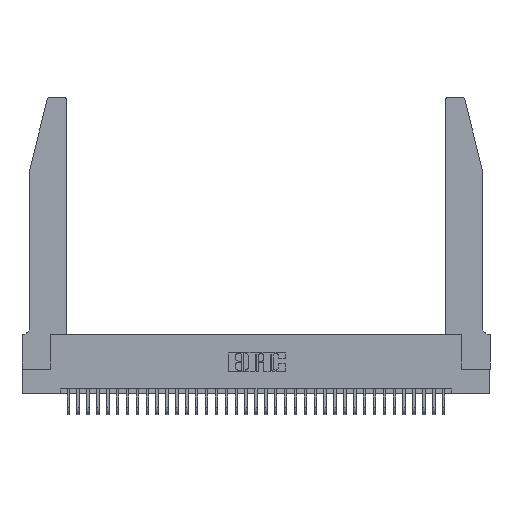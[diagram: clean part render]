
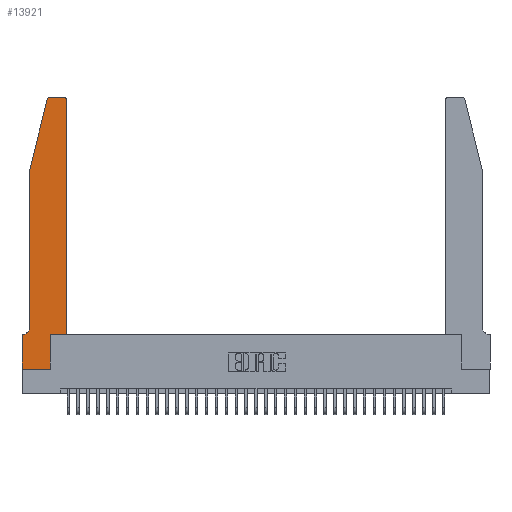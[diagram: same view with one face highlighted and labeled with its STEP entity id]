
A CAD part, top view. The second image highlights one B-rep face of the part: STEP entity #13921.
In plain terms, the highlighted planar face has unit normal (0, 0, 1).
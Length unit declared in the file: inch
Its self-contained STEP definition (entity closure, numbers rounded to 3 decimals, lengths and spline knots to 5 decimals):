
#809 = CARTESIAN_POINT ( 'NONE',  ( 0.284, 2.75, 0.37 ) ) ;
#862 = DIRECTION ( 'NONE',  ( -1., 0., 0. ) ) ;
#1771 = AXIS2_PLACEMENT_3D ( 'NONE', #9442, #9686, #862 ) ;
#2038 = EDGE_CURVE ( 'NONE', #28703, #14922, #35239, .T. ) ;
#2116 = DIRECTION ( 'NONE',  ( 0., -1., 0. ) ) ;
#2224 = DIRECTION ( 'NONE',  ( 1., 0., 0. ) ) ;
#2699 = CARTESIAN_POINT ( 'NONE',  ( 0.4505, 0.35, 0.37 ) ) ;
#2834 = CARTESIAN_POINT ( 'NONE',  ( 0.4505, 0.35, 0.37 ) ) ;
#3368 = EDGE_CURVE ( 'NONE', #25652, #6216, #4881, .T. ) ;
#3410 = VECTOR ( 'NONE', #4478, 39.37008 ) ;
#3908 = PLANE ( 'NONE',  #33992 ) ;
#4478 = DIRECTION ( 'NONE',  ( 0., -1., 0. ) ) ;
#4808 = EDGE_CURVE ( 'NONE', #6216, #18224, #8811, .T. ) ;
#4881 = LINE ( 'NONE', #33377, #10273 ) ;
#5211 = CARTESIAN_POINT ( 'NONE',  ( 0., 0., 0.37 ) ) ;
#5376 = ORIENTED_EDGE ( 'NONE', *, *, #4808, .T. ) ;
#5624 = ORIENTED_EDGE ( 'NONE', *, *, #27006, .T. ) ;
#5787 = EDGE_CURVE ( 'NONE', #14922, #32953, #15535, .T. ) ;
#5981 = EDGE_CURVE ( 'NONE', #8327, #28703, #29503, .T. ) ;
#6216 = VERTEX_POINT ( 'NONE', #22703 ) ;
#6355 = LINE ( 'NONE', #8183, #35257 ) ;
#6808 = DIRECTION ( 'NONE',  ( 0., 0., 1. ) ) ;
#7999 = AXIS2_PLACEMENT_3D ( 'NONE', #19519, #10666, #2224 ) ;
#8140 = EDGE_CURVE ( 'NONE', #12498, #15080, #6355, .T. ) ;
#8149 = ORIENTED_EDGE ( 'NONE', *, *, #17963, .T. ) ;
#8183 = CARTESIAN_POINT ( 'NONE',  ( 0.0755, 2., 0.37 ) ) ;
#8206 = VECTOR ( 'NONE', #22897, 39.37008 ) ;
#8327 = VERTEX_POINT ( 'NONE', #27650 ) ;
#8572 = EDGE_CURVE ( 'NONE', #32953, #13648, #10065, .T. ) ;
#8811 = LINE ( 'NONE', #28832, #3410 ) ;
#9442 = CARTESIAN_POINT ( 'NONE',  ( 0.0055, 0.42, 0.37 ) ) ;
#9642 = CARTESIAN_POINT ( 'NONE',  ( 0.4205, 2.75, 0.37 ) ) ;
#9686 = DIRECTION ( 'NONE',  ( 0., 0., -1. ) ) ;
#10065 = CIRCLE ( 'NONE', #18178, 0.03 ) ;
#10095 = VECTOR ( 'NONE', #31358, 39.37008 ) ;
#10106 = CARTESIAN_POINT ( 'NONE',  ( 0.25487, 2.72718, 0.37 ) ) ;
#10134 = CARTESIAN_POINT ( 'NONE',  ( 0.0755, 0.42, 0.37 ) ) ;
#10273 = VECTOR ( 'NONE', #13148, 39.37008 ) ;
#10666 = DIRECTION ( 'NONE',  ( 0., 0., 1. ) ) ;
#10726 = DIRECTION ( 'NONE',  ( 1., 0., 0. ) ) ;
#11083 = CARTESIAN_POINT ( 'NONE',  ( 0.4505, 2.72, 0.37 ) ) ;
#11756 = ORIENTED_EDGE ( 'NONE', *, *, #35417, .T. ) ;
#11978 = CARTESIAN_POINT ( 'NONE',  ( 0.0055, 0.35, 0.37 ) ) ;
#12498 = VERTEX_POINT ( 'NONE', #28079 ) ;
#13148 = DIRECTION ( 'NONE',  ( -1., 0., 0. ) ) ;
#13308 = DIRECTION ( 'NONE',  ( 0., 1., 0. ) ) ;
#13494 = ORIENTED_EDGE ( 'NONE', *, *, #34876, .T. ) ;
#13648 = VERTEX_POINT ( 'NONE', #10106 ) ;
#13921 = ADVANCED_FACE ( 'NONE', ( #33702 ), #3908, .T. ) ;
#14227 = VECTOR ( 'NONE', #28774, 39.37008 ) ;
#14266 = ORIENTED_EDGE ( 'NONE', *, *, #5981, .T. ) ;
#14922 = VERTEX_POINT ( 'NONE', #9642 ) ;
#15080 = VERTEX_POINT ( 'NONE', #10134 ) ;
#15535 = LINE ( 'NONE', #16191, #14227 ) ;
#16191 = CARTESIAN_POINT ( 'NONE',  ( 0.2605, 2.75, 0.37 ) ) ;
#16517 = CIRCLE ( 'NONE', #1771, 0.07 ) ;
#16568 = ORIENTED_EDGE ( 'NONE', *, *, #8572, .T. ) ;
#16888 = LINE ( 'NONE', #18867, #34554 ) ;
#17651 = EDGE_LOOP ( 'NONE', ( #35741, #16568, #5624, #27489, #8149, #18265, #5376, #11756, #31262, #13494, #14266, #31800 ) ) ;
#17836 = LINE ( 'NONE', #5211, #23734 ) ;
#17963 = EDGE_CURVE ( 'NONE', #15080, #25652, #16517, .T. ) ;
#18178 = AXIS2_PLACEMENT_3D ( 'NONE', #35896, #21997, #24482 ) ;
#18224 = VERTEX_POINT ( 'NONE', #19372 ) ;
#18265 = ORIENTED_EDGE ( 'NONE', *, *, #3368, .T. ) ;
#18867 = CARTESIAN_POINT ( 'NONE',  ( 0.2865, 0.35, 0.37 ) ) ;
#19372 = CARTESIAN_POINT ( 'NONE',  ( 0., 0., 0.37 ) ) ;
#19519 = CARTESIAN_POINT ( 'NONE',  ( 0.4205, 2.72, 0.37 ) ) ;
#20144 = LINE ( 'NONE', #21647, #23264 ) ;
#21647 = CARTESIAN_POINT ( 'NONE',  ( 0.0755, 2., 0.37 ) ) ;
#21714 = CARTESIAN_POINT ( 'NONE',  ( 0., 0.35, 0.37 ) ) ;
#21997 = DIRECTION ( 'NONE',  ( 0., 0., 1. ) ) ;
#22198 = LINE ( 'NONE', #2699, #8206 ) ;
#22703 = CARTESIAN_POINT ( 'NONE',  ( 0., 0.35, 0.37 ) ) ;
#22897 = DIRECTION ( 'NONE',  ( 1., 0., 0. ) ) ;
#23264 = VECTOR ( 'NONE', #36075, 39.37008 ) ;
#23734 = VECTOR ( 'NONE', #10726, 39.37008 ) ;
#24077 = DIRECTION ( 'NONE',  ( 1., 0., 0. ) ) ;
#24482 = DIRECTION ( 'NONE',  ( 1., 0., 0. ) ) ;
#25652 = VERTEX_POINT ( 'NONE', #11978 ) ;
#27006 = EDGE_CURVE ( 'NONE', #13648, #12498, #20144, .T. ) ;
#27196 = VERTEX_POINT ( 'NONE', #37085 ) ;
#27489 = ORIENTED_EDGE ( 'NONE', *, *, #8140, .T. ) ;
#27650 = CARTESIAN_POINT ( 'NONE',  ( 0.4505, 0.35, 0.37 ) ) ;
#28079 = CARTESIAN_POINT ( 'NONE',  ( 0.0755, 2., 0.37 ) ) ;
#28703 = VERTEX_POINT ( 'NONE', #11083 ) ;
#28774 = DIRECTION ( 'NONE',  ( -1., 0., 0. ) ) ;
#28832 = CARTESIAN_POINT ( 'NONE',  ( 0., 0., 0.37 ) ) ;
#29503 = LINE ( 'NONE', #2834, #10095 ) ;
#31262 = ORIENTED_EDGE ( 'NONE', *, *, #36758, .T. ) ;
#31358 = DIRECTION ( 'NONE',  ( 0., 1., 0. ) ) ;
#31800 = ORIENTED_EDGE ( 'NONE', *, *, #2038, .T. ) ;
#32953 = VERTEX_POINT ( 'NONE', #809 ) ;
#33377 = CARTESIAN_POINT ( 'NONE',  ( 0.0755, 0.35, 0.37 ) ) ;
#33702 = FACE_OUTER_BOUND ( 'NONE', #17651, .T. ) ;
#33992 = AXIS2_PLACEMENT_3D ( 'NONE', #21714, #6808, #24077 ) ;
#34554 = VECTOR ( 'NONE', #13308, 39.37008 ) ;
#34876 = EDGE_CURVE ( 'NONE', #27196, #8327, #22198, .T. ) ;
#34932 = CARTESIAN_POINT ( 'NONE',  ( 0.2865, 0., 0.37 ) ) ;
#35239 = CIRCLE ( 'NONE', #7999, 0.03 ) ;
#35257 = VECTOR ( 'NONE', #2116, 39.37008 ) ;
#35417 = EDGE_CURVE ( 'NONE', #18224, #37218, #17836, .T. ) ;
#35741 = ORIENTED_EDGE ( 'NONE', *, *, #5787, .T. ) ;
#35896 = CARTESIAN_POINT ( 'NONE',  ( 0.284, 2.72, 0.37 ) ) ;
#36075 = DIRECTION ( 'NONE',  ( -0.239, -0.971, 0. ) ) ;
#36758 = EDGE_CURVE ( 'NONE', #37218, #27196, #16888, .T. ) ;
#37085 = CARTESIAN_POINT ( 'NONE',  ( 0.2865, 0.35, 0.37 ) ) ;
#37218 = VERTEX_POINT ( 'NONE', #34932 ) ;
